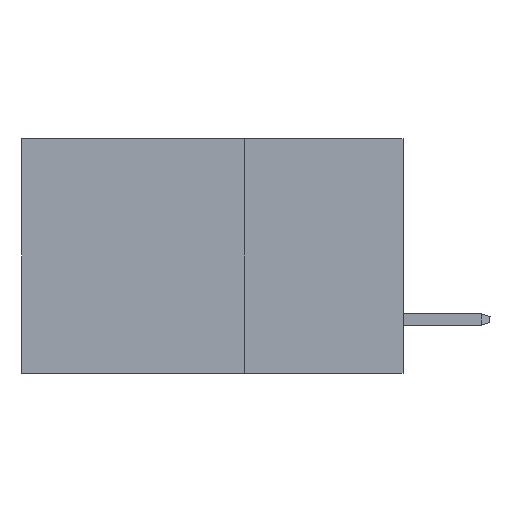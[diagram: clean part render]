
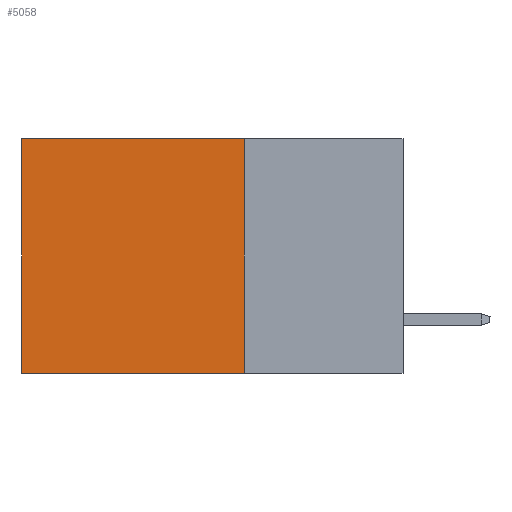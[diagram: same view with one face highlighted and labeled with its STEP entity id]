
A CAD part, left-side view. The second image highlights one B-rep face of the part: STEP entity #5058.
In plain terms, the highlighted planar face has unit normal (-1, 0, 0).
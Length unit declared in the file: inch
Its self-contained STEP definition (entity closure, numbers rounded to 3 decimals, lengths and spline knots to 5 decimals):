
#76 = VERTEX_POINT ( 'NONE', #16371 ) ;
#478 = EDGE_CURVE ( 'NONE', #21141, #725, #2975, .T. ) ;
#725 = VERTEX_POINT ( 'NONE', #19258 ) ;
#853 = PLANE ( 'NONE',  #16923 ) ;
#2255 = VECTOR ( 'NONE', #11905, 39.37008 ) ;
#2838 = DIRECTION ( 'NONE',  ( 0., 0., -1. ) ) ;
#2899 = EDGE_LOOP ( 'NONE', ( #21556, #11796, #16794, #4459 ) ) ;
#2975 = LINE ( 'NONE', #18398, #2255 ) ;
#4417 = VECTOR ( 'NONE', #17174, 39.37008 ) ;
#4459 = ORIENTED_EDGE ( 'NONE', *, *, #478, .T. ) ;
#4600 = FACE_OUTER_BOUND ( 'NONE', #2899, .T. ) ;
#5058 = ADVANCED_FACE ( 'NONE', ( #4600 ), #853, .F. ) ;
#7017 = VERTEX_POINT ( 'NONE', #18710 ) ;
#7366 = LINE ( 'NONE', #17399, #4417 ) ;
#8369 = VECTOR ( 'NONE', #21570, 39.37008 ) ;
#9470 = DIRECTION ( 'NONE',  ( 1., 0., 0. ) ) ;
#9686 = CARTESIAN_POINT ( 'NONE',  ( 0.2875, 0.6, 0. ) ) ;
#10628 = EDGE_CURVE ( 'NONE', #21141, #76, #14121, .T. ) ;
#10933 = EDGE_CURVE ( 'NONE', #76, #7017, #7366, .T. ) ;
#11496 = CARTESIAN_POINT ( 'NONE',  ( 0.2875, 0.25, 0. ) ) ;
#11796 = ORIENTED_EDGE ( 'NONE', *, *, #10933, .F. ) ;
#11905 = DIRECTION ( 'NONE',  ( 0., 1., 0. ) ) ;
#13633 = EDGE_CURVE ( 'NONE', #725, #7017, #16504, .T. ) ;
#14121 = LINE ( 'NONE', #20815, #21111 ) ;
#14339 = DIRECTION ( 'NONE',  ( 0., 0., -1. ) ) ;
#16371 = CARTESIAN_POINT ( 'NONE',  ( 0.2875, 0.25, -0.37 ) ) ;
#16504 = LINE ( 'NONE', #9686, #8369 ) ;
#16794 = ORIENTED_EDGE ( 'NONE', *, *, #10628, .F. ) ;
#16923 = AXIS2_PLACEMENT_3D ( 'NONE', #21249, #9470, #2838 ) ;
#17174 = DIRECTION ( 'NONE',  ( 0., 1., 0. ) ) ;
#17399 = CARTESIAN_POINT ( 'NONE',  ( 0.2875, 0.25, -0.37 ) ) ;
#18398 = CARTESIAN_POINT ( 'NONE',  ( 0.2875, 0.25, 0. ) ) ;
#18710 = CARTESIAN_POINT ( 'NONE',  ( 0.2875, 0.6, -0.37 ) ) ;
#19258 = CARTESIAN_POINT ( 'NONE',  ( 0.2875, 0.6, 0. ) ) ;
#20815 = CARTESIAN_POINT ( 'NONE',  ( 0.2875, 0.25, 0. ) ) ;
#21111 = VECTOR ( 'NONE', #14339, 39.37008 ) ;
#21141 = VERTEX_POINT ( 'NONE', #11496 ) ;
#21249 = CARTESIAN_POINT ( 'NONE',  ( 0.2875, 0.25, 0. ) ) ;
#21556 = ORIENTED_EDGE ( 'NONE', *, *, #13633, .T. ) ;
#21570 = DIRECTION ( 'NONE',  ( 0., 0., -1. ) ) ;
